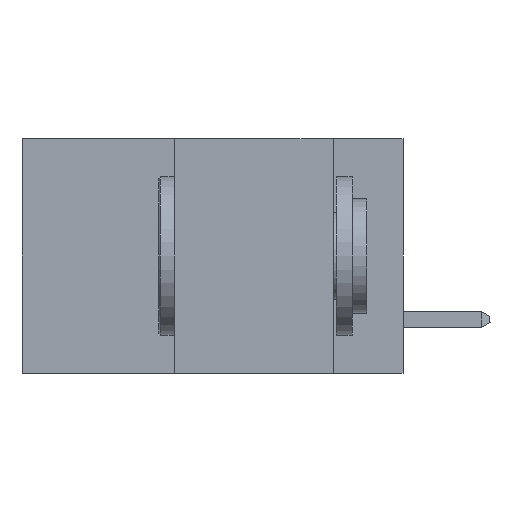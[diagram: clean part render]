
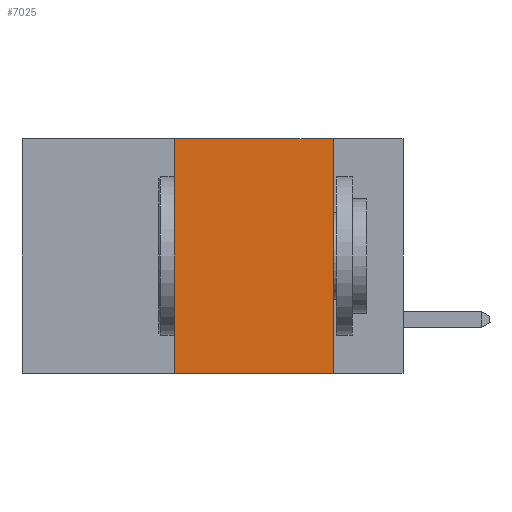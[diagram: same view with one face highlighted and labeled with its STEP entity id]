
A CAD part, left-side view. The second image highlights one B-rep face of the part: STEP entity #7025.
In plain terms, the highlighted planar face has unit normal (-1, 0, 0).
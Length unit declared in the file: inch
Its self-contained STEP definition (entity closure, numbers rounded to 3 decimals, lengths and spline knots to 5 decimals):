
#9 = CARTESIAN_POINT ( 'NONE',  ( 0., 0.11, -0.37 ) ) ;
#99 = EDGE_CURVE ( 'NONE', #8299, #16111, #15278, .T. ) ;
#472 = VECTOR ( 'NONE', #11239, 39.37008 ) ;
#959 = AXIS2_PLACEMENT_3D ( 'NONE', #5083, #15236, #6554 ) ;
#983 = LINE ( 'NONE', #9801, #472 ) ;
#2101 = CARTESIAN_POINT ( 'NONE',  ( 0., 0.36, -0.37 ) ) ;
#4164 = CARTESIAN_POINT ( 'NONE',  ( 0., 0.36, 0. ) ) ;
#4830 = VERTEX_POINT ( 'NONE', #2101 ) ;
#5083 = CARTESIAN_POINT ( 'NONE',  ( 0., 0.6, 0. ) ) ;
#6554 = DIRECTION ( 'NONE',  ( 0., 0., -1. ) ) ;
#6814 = DIRECTION ( 'NONE',  ( 0., -1., 0. ) ) ;
#7025 = ADVANCED_FACE ( 'NONE', ( #9332 ), #12299, .F. ) ;
#8299 = VERTEX_POINT ( 'NONE', #12317 ) ;
#9241 = ORIENTED_EDGE ( 'NONE', *, *, #99, .F. ) ;
#9316 = ORIENTED_EDGE ( 'NONE', *, *, #10781, .F. ) ;
#9332 = FACE_OUTER_BOUND ( 'NONE', #18359, .T. ) ;
#9801 = CARTESIAN_POINT ( 'NONE',  ( 0., 0.36, 0. ) ) ;
#10686 = VECTOR ( 'NONE', #6814, 39.37008 ) ;
#10781 = EDGE_CURVE ( 'NONE', #4830, #16561, #983, .T. ) ;
#11134 = CARTESIAN_POINT ( 'NONE',  ( 0., 0.6, -0.37 ) ) ;
#11239 = DIRECTION ( 'NONE',  ( 0., 0., 1. ) ) ;
#11284 = EDGE_CURVE ( 'NONE', #16561, #8299, #18830, .T. ) ;
#12299 = PLANE ( 'NONE',  #959 ) ;
#12317 = CARTESIAN_POINT ( 'NONE',  ( 0., 0.11, 0. ) ) ;
#12921 = DIRECTION ( 'NONE',  ( 0., 0., -1. ) ) ;
#13105 = CARTESIAN_POINT ( 'NONE',  ( 0., 0.11, 0. ) ) ;
#14003 = ORIENTED_EDGE ( 'NONE', *, *, #11284, .F. ) ;
#14393 = VECTOR ( 'NONE', #12921, 39.37008 ) ;
#14534 = LINE ( 'NONE', #11134, #10686 ) ;
#14949 = ORIENTED_EDGE ( 'NONE', *, *, #15252, .T. ) ;
#15056 = CARTESIAN_POINT ( 'NONE',  ( 0., 0.6, 0. ) ) ;
#15150 = VECTOR ( 'NONE', #16429, 39.37008 ) ;
#15236 = DIRECTION ( 'NONE',  ( 1., 0., 0. ) ) ;
#15252 = EDGE_CURVE ( 'NONE', #4830, #16111, #14534, .T. ) ;
#15278 = LINE ( 'NONE', #13105, #14393 ) ;
#16111 = VERTEX_POINT ( 'NONE', #9 ) ;
#16429 = DIRECTION ( 'NONE',  ( 0., -1., 0. ) ) ;
#16561 = VERTEX_POINT ( 'NONE', #4164 ) ;
#18359 = EDGE_LOOP ( 'NONE', ( #9241, #14003, #9316, #14949 ) ) ;
#18830 = LINE ( 'NONE', #15056, #15150 ) ;
